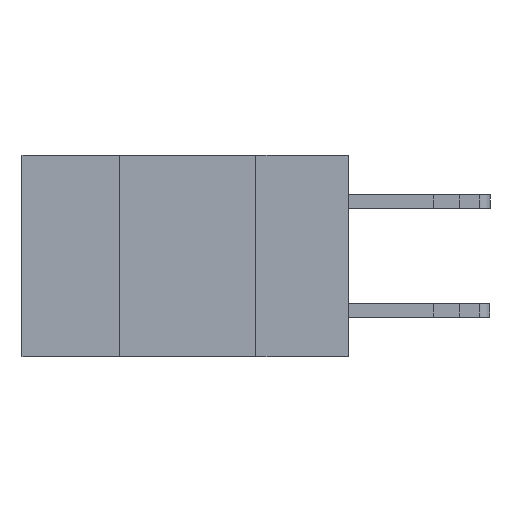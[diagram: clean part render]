
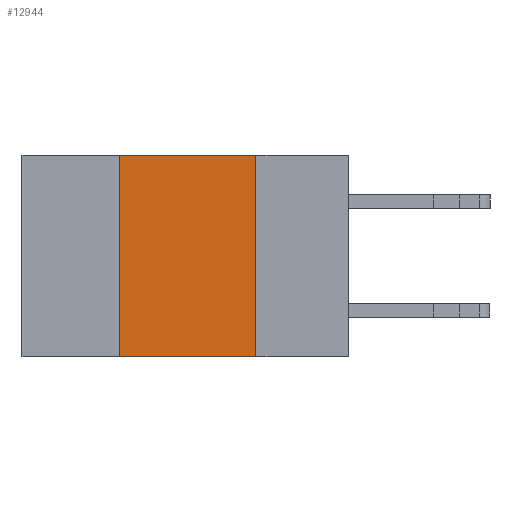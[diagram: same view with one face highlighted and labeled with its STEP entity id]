
A CAD part, left-side view. The second image highlights one B-rep face of the part: STEP entity #12944.
In plain terms, the highlighted planar face has unit normal (-1, 0, 0).
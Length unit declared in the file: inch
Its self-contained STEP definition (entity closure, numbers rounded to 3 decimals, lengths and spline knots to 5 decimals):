
#389 = VECTOR ( 'NONE', #5642, 39.37008 ) ;
#694 = DIRECTION ( 'NONE',  ( 0., -1., 0. ) ) ;
#963 = VECTOR ( 'NONE', #694, 39.37008 ) ;
#1461 = ORIENTED_EDGE ( 'NONE', *, *, #12571, .F. ) ;
#1679 = VERTEX_POINT ( 'NONE', #10238 ) ;
#1685 = CARTESIAN_POINT ( 'NONE',  ( 0., 0.42, 0. ) ) ;
#2507 = ORIENTED_EDGE ( 'NONE', *, *, #11900, .T. ) ;
#2928 = CARTESIAN_POINT ( 'NONE',  ( 0., 0.6, 0. ) ) ;
#2932 = CARTESIAN_POINT ( 'NONE',  ( 0., 0.17, -0.37 ) ) ;
#3491 = PLANE ( 'NONE',  #9482 ) ;
#3535 = VERTEX_POINT ( 'NONE', #9778 ) ;
#3901 = LINE ( 'NONE', #2928, #963 ) ;
#4493 = LINE ( 'NONE', #1685, #12268 ) ;
#4531 = VERTEX_POINT ( 'NONE', #2932 ) ;
#4562 = DIRECTION ( 'NONE',  ( 1., 0., 0. ) ) ;
#4669 = LINE ( 'NONE', #4972, #12774 ) ;
#4808 = FACE_OUTER_BOUND ( 'NONE', #5760, .T. ) ;
#4972 = CARTESIAN_POINT ( 'NONE',  ( 0., 0.6, -0.37 ) ) ;
#5642 = DIRECTION ( 'NONE',  ( 0., 0., -1. ) ) ;
#5760 = EDGE_LOOP ( 'NONE', ( #9679, #12646, #1461, #2507 ) ) ;
#6868 = LINE ( 'NONE', #7702, #389 ) ;
#7702 = CARTESIAN_POINT ( 'NONE',  ( 0., 0.17, 0. ) ) ;
#8090 = CARTESIAN_POINT ( 'NONE',  ( 0., 0.42, -0.37 ) ) ;
#8672 = EDGE_CURVE ( 'NONE', #1679, #3535, #3901, .T. ) ;
#9482 = AXIS2_PLACEMENT_3D ( 'NONE', #10939, #4562, #11988 ) ;
#9679 = ORIENTED_EDGE ( 'NONE', *, *, #11559, .F. ) ;
#9778 = CARTESIAN_POINT ( 'NONE',  ( 0., 0.17, 0. ) ) ;
#10238 = CARTESIAN_POINT ( 'NONE',  ( 0., 0.42, 0. ) ) ;
#10250 = DIRECTION ( 'NONE',  ( 0., -1., 0. ) ) ;
#10939 = CARTESIAN_POINT ( 'NONE',  ( 0., 0.6, 0. ) ) ;
#11141 = VERTEX_POINT ( 'NONE', #8090 ) ;
#11559 = EDGE_CURVE ( 'NONE', #3535, #4531, #6868, .T. ) ;
#11900 = EDGE_CURVE ( 'NONE', #11141, #4531, #4669, .T. ) ;
#11988 = DIRECTION ( 'NONE',  ( 0., 0., -1. ) ) ;
#12268 = VECTOR ( 'NONE', #12392, 39.37008 ) ;
#12392 = DIRECTION ( 'NONE',  ( 0., 0., 1. ) ) ;
#12571 = EDGE_CURVE ( 'NONE', #11141, #1679, #4493, .T. ) ;
#12646 = ORIENTED_EDGE ( 'NONE', *, *, #8672, .F. ) ;
#12774 = VECTOR ( 'NONE', #10250, 39.37008 ) ;
#12944 = ADVANCED_FACE ( 'NONE', ( #4808 ), #3491, .F. ) ;
